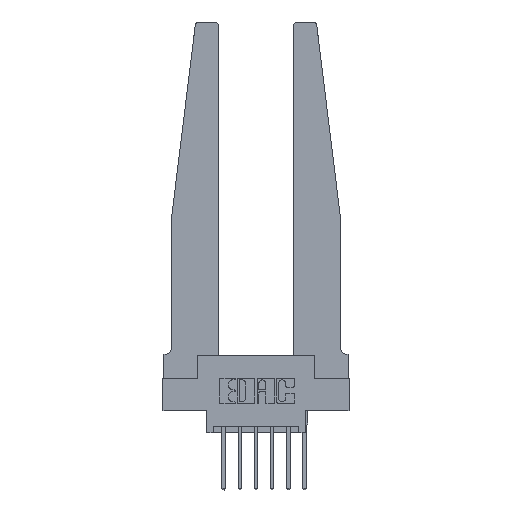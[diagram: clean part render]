
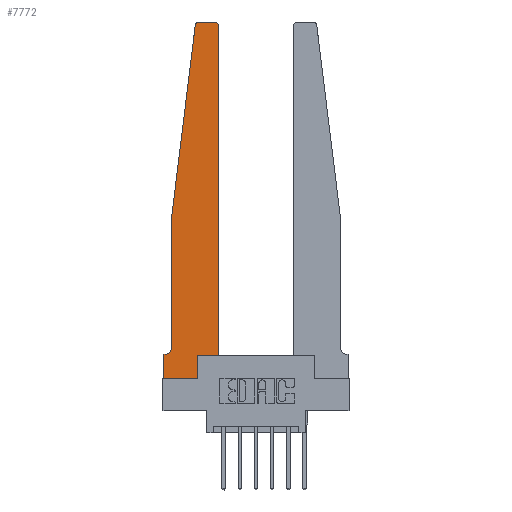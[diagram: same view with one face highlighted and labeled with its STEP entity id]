
A CAD part, top view. The second image highlights one B-rep face of the part: STEP entity #7772.
In plain terms, the highlighted planar face has unit normal (0, 0, 1).
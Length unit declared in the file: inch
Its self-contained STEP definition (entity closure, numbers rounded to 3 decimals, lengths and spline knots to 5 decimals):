
#80 = EDGE_CURVE ( 'NONE', #2780, #13030, #13191, .T. ) ;
#206 = CARTESIAN_POINT ( 'NONE',  ( 0.065, 0.2375, 0.37 ) ) ;
#281 = EDGE_CURVE ( 'NONE', #8138, #1601, #13305, .T. ) ;
#416 = VECTOR ( 'NONE', #10471, 39.37008 ) ;
#909 = VERTEX_POINT ( 'NONE', #5289 ) ;
#1008 = ORIENTED_EDGE ( 'NONE', *, *, #5494, .T. ) ;
#1104 = CARTESIAN_POINT ( 'NONE',  ( 0., 0.1875, 0.37 ) ) ;
#1205 = CARTESIAN_POINT ( 'NONE',  ( 0.425, 2.72, 0.37 ) ) ;
#1278 = VECTOR ( 'NONE', #7827, 39.37008 ) ;
#1601 = VERTEX_POINT ( 'NONE', #1205 ) ;
#1636 = LINE ( 'NONE', #13504, #11931 ) ;
#1782 = ORIENTED_EDGE ( 'NONE', *, *, #13365, .T. ) ;
#1851 = DIRECTION ( 'NONE',  ( 0., -1., 0. ) ) ;
#1907 = LINE ( 'NONE', #12402, #416 ) ;
#2513 = CIRCLE ( 'NONE', #9768, 0.03 ) ;
#2565 = EDGE_CURVE ( 'NONE', #3802, #7401, #2843, .T. ) ;
#2592 = EDGE_CURVE ( 'NONE', #13030, #3802, #2716, .T. ) ;
#2716 = LINE ( 'NONE', #7046, #6755 ) ;
#2748 = LINE ( 'NONE', #10042, #12081 ) ;
#2777 = DIRECTION ( 'NONE',  ( -1., 0., 0. ) ) ;
#2780 = VERTEX_POINT ( 'NONE', #11980 ) ;
#2784 = ORIENTED_EDGE ( 'NONE', *, *, #2565, .T. ) ;
#2843 = LINE ( 'NONE', #7947, #1278 ) ;
#2945 = DIRECTION ( 'NONE',  ( -1., 0., 0. ) ) ;
#3205 = ORIENTED_EDGE ( 'NONE', *, *, #10573, .T. ) ;
#3672 = CARTESIAN_POINT ( 'NONE',  ( 0., 0.1875, 0.37 ) ) ;
#3696 = ORIENTED_EDGE ( 'NONE', *, *, #2592, .T. ) ;
#3802 = VERTEX_POINT ( 'NONE', #7058 ) ;
#4007 = DIRECTION ( 'NONE',  ( 0., 0., -1. ) ) ;
#4257 = AXIS2_PLACEMENT_3D ( 'NONE', #6016, #4007, #2777 ) ;
#4580 = VERTEX_POINT ( 'NONE', #6754 ) ;
#4848 = AXIS2_PLACEMENT_3D ( 'NONE', #1104, #12616, #8530 ) ;
#4920 = DIRECTION ( 'NONE',  ( 1., 0., 0. ) ) ;
#4923 = CARTESIAN_POINT ( 'NONE',  ( 0.015, 0.1875, 0.37 ) ) ;
#5215 = CARTESIAN_POINT ( 'NONE',  ( 0.25, 2.75, 0.37 ) ) ;
#5289 = CARTESIAN_POINT ( 'NONE',  ( 0.2605, 0.18, 0.37 ) ) ;
#5494 = EDGE_CURVE ( 'NONE', #7401, #6882, #12855, .T. ) ;
#5790 = VECTOR ( 'NONE', #1851, 39.37008 ) ;
#5887 = VERTEX_POINT ( 'NONE', #6136 ) ;
#6008 = EDGE_CURVE ( 'NONE', #1601, #4580, #2513, .T. ) ;
#6016 = CARTESIAN_POINT ( 'NONE',  ( 0.015, 0.2375, 0.37 ) ) ;
#6025 = VECTOR ( 'NONE', #2945, 39.37008 ) ;
#6114 = DIRECTION ( 'NONE',  ( -1., 0., 0. ) ) ;
#6136 = CARTESIAN_POINT ( 'NONE',  ( 0.2605, 0., 0.37 ) ) ;
#6726 = DIRECTION ( 'NONE',  ( 0., 1., 0. ) ) ;
#6754 = CARTESIAN_POINT ( 'NONE',  ( 0.395, 2.75, 0.37 ) ) ;
#6755 = VECTOR ( 'NONE', #6772, 39.37008 ) ;
#6772 = DIRECTION ( 'NONE',  ( -0.122, -0.992, 0. ) ) ;
#6779 = DIRECTION ( 'NONE',  ( 0., 0., 1. ) ) ;
#6882 = VERTEX_POINT ( 'NONE', #4923 ) ;
#7046 = CARTESIAN_POINT ( 'NONE',  ( 0.065, 1.25, 0.37 ) ) ;
#7058 = CARTESIAN_POINT ( 'NONE',  ( 0.065, 1.25, 0.37 ) ) ;
#7069 = CARTESIAN_POINT ( 'NONE',  ( 0.065, 0.1875, 0.37 ) ) ;
#7347 = CARTESIAN_POINT ( 'NONE',  ( 0.425, 0.18, 0.37 ) ) ;
#7366 = CARTESIAN_POINT ( 'NONE',  ( 0., 0., 0.37 ) ) ;
#7401 = VERTEX_POINT ( 'NONE', #206 ) ;
#7772 = ADVANCED_FACE ( 'NONE', ( #8389 ), #9622, .T. ) ;
#7827 = DIRECTION ( 'NONE',  ( 0., -1., 0. ) ) ;
#7911 = EDGE_CURVE ( 'NONE', #13515, #5887, #1636, .T. ) ;
#7947 = CARTESIAN_POINT ( 'NONE',  ( 0.065, 1.25, 0.37 ) ) ;
#7971 = CARTESIAN_POINT ( 'NONE',  ( 0.425, 0.18, 0.37 ) ) ;
#8138 = VERTEX_POINT ( 'NONE', #7347 ) ;
#8389 = FACE_OUTER_BOUND ( 'NONE', #9796, .T. ) ;
#8425 = VECTOR ( 'NONE', #6114, 39.37008 ) ;
#8530 = DIRECTION ( 'NONE',  ( 1., 0., 0. ) ) ;
#8775 = AXIS2_PLACEMENT_3D ( 'NONE', #8862, #6779, #11179 ) ;
#8837 = ORIENTED_EDGE ( 'NONE', *, *, #6008, .T. ) ;
#8862 = CARTESIAN_POINT ( 'NONE',  ( 0.27653, 2.72, 0.37 ) ) ;
#9168 = LINE ( 'NONE', #11364, #5790 ) ;
#9203 = ORIENTED_EDGE ( 'NONE', *, *, #7911, .T. ) ;
#9236 = DIRECTION ( 'NONE',  ( 1., 0., 0. ) ) ;
#9429 = VECTOR ( 'NONE', #6726, 39.37008 ) ;
#9622 = PLANE ( 'NONE',  #4848 ) ;
#9768 = AXIS2_PLACEMENT_3D ( 'NONE', #11301, #10264, #9236 ) ;
#9796 = EDGE_LOOP ( 'NONE', ( #11835, #12914, #3696, #2784, #1008, #13659, #3205, #9203, #13404, #1782, #11586, #8837 ) ) ;
#9976 = DIRECTION ( 'NONE',  ( 1., 0., 0. ) ) ;
#10042 = CARTESIAN_POINT ( 'NONE',  ( 0.425, 0.18, 0.37 ) ) ;
#10264 = DIRECTION ( 'NONE',  ( 0., 0., 1. ) ) ;
#10471 = DIRECTION ( 'NONE',  ( 0., 1., 0. ) ) ;
#10573 = EDGE_CURVE ( 'NONE', #13039, #13515, #9168, .T. ) ;
#10941 = EDGE_CURVE ( 'NONE', #6882, #13039, #11348, .T. ) ;
#11179 = DIRECTION ( 'NONE',  ( 1., 0., 0. ) ) ;
#11301 = CARTESIAN_POINT ( 'NONE',  ( 0.395, 2.72, 0.37 ) ) ;
#11348 = LINE ( 'NONE', #7069, #8425 ) ;
#11364 = CARTESIAN_POINT ( 'NONE',  ( 0., 0., 0.37 ) ) ;
#11586 = ORIENTED_EDGE ( 'NONE', *, *, #281, .T. ) ;
#11835 = ORIENTED_EDGE ( 'NONE', *, *, #12243, .T. ) ;
#11931 = VECTOR ( 'NONE', #4920, 39.37008 ) ;
#11980 = CARTESIAN_POINT ( 'NONE',  ( 0.27653, 2.75, 0.37 ) ) ;
#12030 = CARTESIAN_POINT ( 'NONE',  ( 0.24675, 2.72367, 0.37 ) ) ;
#12081 = VECTOR ( 'NONE', #9976, 39.37008 ) ;
#12243 = EDGE_CURVE ( 'NONE', #4580, #2780, #13521, .T. ) ;
#12402 = CARTESIAN_POINT ( 'NONE',  ( 0.2605, 0.18, 0.37 ) ) ;
#12616 = DIRECTION ( 'NONE',  ( 0., 0., 1. ) ) ;
#12855 = CIRCLE ( 'NONE', #4257, 0.05 ) ;
#12914 = ORIENTED_EDGE ( 'NONE', *, *, #80, .T. ) ;
#13030 = VERTEX_POINT ( 'NONE', #12030 ) ;
#13039 = VERTEX_POINT ( 'NONE', #3672 ) ;
#13191 = CIRCLE ( 'NONE', #8775, 0.03 ) ;
#13305 = LINE ( 'NONE', #7971, #9429 ) ;
#13365 = EDGE_CURVE ( 'NONE', #909, #8138, #2748, .T. ) ;
#13404 = ORIENTED_EDGE ( 'NONE', *, *, #13428, .T. ) ;
#13428 = EDGE_CURVE ( 'NONE', #5887, #909, #1907, .T. ) ;
#13504 = CARTESIAN_POINT ( 'NONE',  ( 0., 0., 0.37 ) ) ;
#13515 = VERTEX_POINT ( 'NONE', #7366 ) ;
#13521 = LINE ( 'NONE', #5215, #6025 ) ;
#13659 = ORIENTED_EDGE ( 'NONE', *, *, #10941, .T. ) ;
